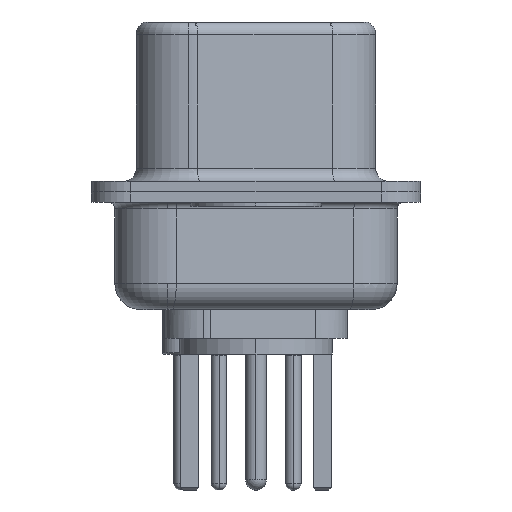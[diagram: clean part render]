
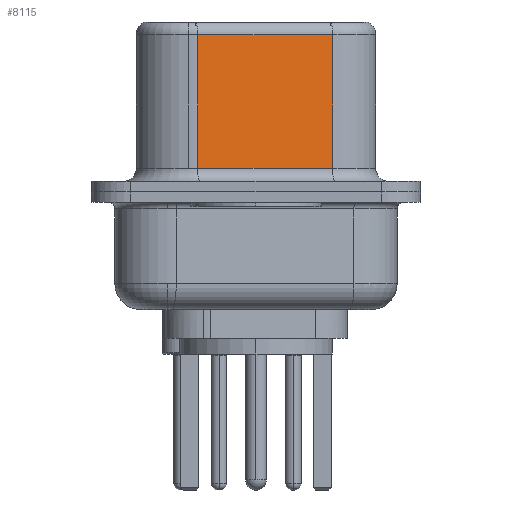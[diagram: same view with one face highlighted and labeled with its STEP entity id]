
A CAD part, left-side view. The second image highlights one B-rep face of the part: STEP entity #8115.
In plain terms, the highlighted planar face has unit normal (-0.985, -0.174, 0).
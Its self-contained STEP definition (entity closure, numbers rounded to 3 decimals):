
#602 = PLANE ( 'NONE',  #14628 ) ;
#1049 = EDGE_LOOP ( 'NONE', ( #1193, #9630, #13995, #5838 ) ) ;
#1193 = ORIENTED_EDGE ( 'NONE', *, *, #16210, .F. ) ;
#2310 = CARTESIAN_POINT ( 'NONE',  ( 3.67, 2.233, 6.02 ) ) ;
#3409 = CARTESIAN_POINT ( 'NONE',  ( 4.58, -2.927, 6.52 ) ) ;
#3736 = VECTOR ( 'NONE', #17011, 1000. ) ;
#5309 = DIRECTION ( 'NONE',  ( -0.174, 0.985, 0. ) ) ;
#5607 = CARTESIAN_POINT ( 'NONE',  ( 4.58, -2.927, 6.02 ) ) ;
#5719 = DIRECTION ( 'NONE',  ( 0.174, -0.985, 0. ) ) ;
#5838 = ORIENTED_EDGE ( 'NONE', *, *, #19512, .T. ) ;
#6684 = VECTOR ( 'NONE', #5309, 1000. ) ;
#6714 = CARTESIAN_POINT ( 'NONE',  ( 4.58, -2.927, 6.52 ) ) ;
#7277 = CARTESIAN_POINT ( 'NONE',  ( 4.58, -2.927, 0.9 ) ) ;
#7373 = LINE ( 'NONE', #15461, #3736 ) ;
#8115 = ADVANCED_FACE ( 'NONE', ( #17054 ), #602, .F. ) ;
#9147 = VECTOR ( 'NONE', #5719, 1000. ) ;
#9630 = ORIENTED_EDGE ( 'NONE', *, *, #16249, .T. ) ;
#10146 = CARTESIAN_POINT ( 'NONE',  ( 4.58, -2.927, 6.02 ) ) ;
#10704 = CARTESIAN_POINT ( 'NONE',  ( 3.67, 2.233, 0.9 ) ) ;
#11040 = LINE ( 'NONE', #10146, #6684 ) ;
#12078 = LINE ( 'NONE', #6714, #20324 ) ;
#12342 = VERTEX_POINT ( 'NONE', #17399 ) ;
#12968 = VERTEX_POINT ( 'NONE', #10704 ) ;
#13498 = LINE ( 'NONE', #7277, #9147 ) ;
#13948 = VERTEX_POINT ( 'NONE', #5607 ) ;
#13995 = ORIENTED_EDGE ( 'NONE', *, *, #18307, .T. ) ;
#14628 = AXIS2_PLACEMENT_3D ( 'NONE', #3409, #20394, #20339 ) ;
#15461 = CARTESIAN_POINT ( 'NONE',  ( 3.67, 2.233, 6.52 ) ) ;
#16210 = EDGE_CURVE ( 'NONE', #13948, #12342, #12078, .T. ) ;
#16249 = EDGE_CURVE ( 'NONE', #13948, #16779, #11040, .T. ) ;
#16779 = VERTEX_POINT ( 'NONE', #2310 ) ;
#17011 = DIRECTION ( 'NONE',  ( 0., 0., -1. ) ) ;
#17054 = FACE_OUTER_BOUND ( 'NONE', #1049, .T. ) ;
#17399 = CARTESIAN_POINT ( 'NONE',  ( 4.58, -2.927, 0.9 ) ) ;
#18184 = DIRECTION ( 'NONE',  ( 0., 0., -1. ) ) ;
#18307 = EDGE_CURVE ( 'NONE', #16779, #12968, #7373, .T. ) ;
#19512 = EDGE_CURVE ( 'NONE', #12968, #12342, #13498, .T. ) ;
#20324 = VECTOR ( 'NONE', #18184, 1000. ) ;
#20339 = DIRECTION ( 'NONE',  ( -0.174, 0.985, 0. ) ) ;
#20394 = DIRECTION ( 'NONE',  ( 0.985, 0.174, 0. ) ) ;
